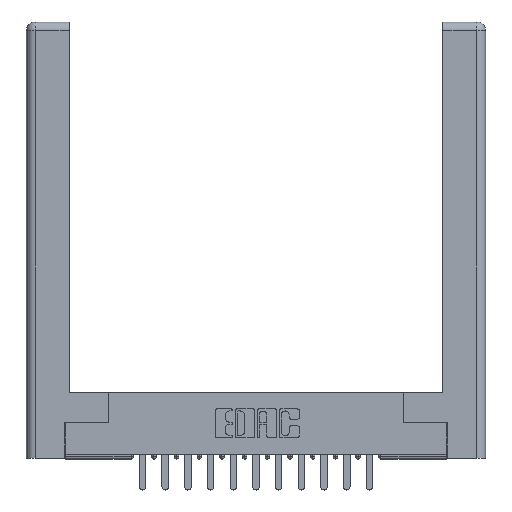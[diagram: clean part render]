
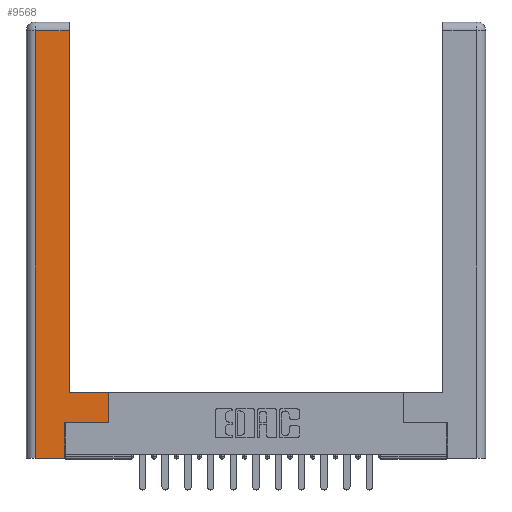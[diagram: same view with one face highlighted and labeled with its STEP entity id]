
A CAD part, top view. The second image highlights one B-rep face of the part: STEP entity #9568.
In plain terms, the highlighted planar face has unit normal (0, 0, 1).
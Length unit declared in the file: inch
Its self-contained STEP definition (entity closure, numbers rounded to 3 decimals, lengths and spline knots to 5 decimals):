
#26 = LINE ( 'NONE', #1676, #1775 ) ;
#109 = VECTOR ( 'NONE', #3716, 39.37008 ) ;
#846 = VERTEX_POINT ( 'NONE', #5462 ) ;
#1676 = CARTESIAN_POINT ( 'NONE',  ( 0.265, 0.245, 0. ) ) ;
#1759 = CARTESIAN_POINT ( 'NONE',  ( 0.565, 0.45, 0. ) ) ;
#1775 = VECTOR ( 'NONE', #3091, 39.37008 ) ;
#1989 = VERTEX_POINT ( 'NONE', #14315 ) ;
#2043 = CARTESIAN_POINT ( 'NONE',  ( 0., 0., 0. ) ) ;
#2630 = LINE ( 'NONE', #7723, #7914 ) ;
#3040 = EDGE_LOOP ( 'NONE', ( #3191, #3085, #13605, #9884, #14091, #15902, #15129, #17615 ) ) ;
#3085 = ORIENTED_EDGE ( 'NONE', *, *, #5495, .T. ) ;
#3091 = DIRECTION ( 'NONE',  ( 0., 1., 0. ) ) ;
#3191 = ORIENTED_EDGE ( 'NONE', *, *, #6668, .T. ) ;
#3481 = VECTOR ( 'NONE', #5031, 39.37008 ) ;
#3716 = DIRECTION ( 'NONE',  ( 0., 1., 0. ) ) ;
#4754 = VECTOR ( 'NONE', #14492, 39.37008 ) ;
#5031 = DIRECTION ( 'NONE',  ( 0., 1., 0. ) ) ;
#5462 = CARTESIAN_POINT ( 'NONE',  ( 0.565, 0.45, 0. ) ) ;
#5495 = EDGE_CURVE ( 'NONE', #13693, #15937, #8516, .T. ) ;
#5678 = LINE ( 'NONE', #1759, #3481 ) ;
#5957 = DIRECTION ( 'NONE',  ( 1., 0., 0. ) ) ;
#6668 = EDGE_CURVE ( 'NONE', #15772, #13693, #15689, .T. ) ;
#6738 = CARTESIAN_POINT ( 'NONE',  ( 0.265, 0., 0. ) ) ;
#7490 = CARTESIAN_POINT ( 'NONE',  ( 0.0615, 2.94, 0. ) ) ;
#7723 = CARTESIAN_POINT ( 'NONE',  ( 0.265, 0., 0. ) ) ;
#7733 = CARTESIAN_POINT ( 'NONE',  ( 0.295, 3., 0. ) ) ;
#7769 = DIRECTION ( 'NONE',  ( 0., 0., -1. ) ) ;
#7914 = VECTOR ( 'NONE', #17553, 39.37008 ) ;
#7922 = CARTESIAN_POINT ( 'NONE',  ( 0.0615, 2.94, 0. ) ) ;
#7933 = VERTEX_POINT ( 'NONE', #6738 ) ;
#8221 = LINE ( 'NONE', #10044, #15889 ) ;
#8516 = LINE ( 'NONE', #7490, #4754 ) ;
#8743 = DIRECTION ( 'NONE',  ( -1., 0., 0. ) ) ;
#9003 = CARTESIAN_POINT ( 'NONE',  ( 0.0615, 0., 0. ) ) ;
#9471 = LINE ( 'NONE', #9003, #13603 ) ;
#9568 = ADVANCED_FACE ( 'NONE', ( #13273 ), #11882, .F. ) ;
#9676 = CARTESIAN_POINT ( 'NONE',  ( 0.0615, 0., 0. ) ) ;
#9677 = VERTEX_POINT ( 'NONE', #16522 ) ;
#9884 = ORIENTED_EDGE ( 'NONE', *, *, #14721, .T. ) ;
#9958 = EDGE_CURVE ( 'NONE', #9677, #1989, #17436, .T. ) ;
#9999 = VECTOR ( 'NONE', #5957, 39.37008 ) ;
#10044 = CARTESIAN_POINT ( 'NONE',  ( 0.295, 0.45, 0. ) ) ;
#10617 = EDGE_CURVE ( 'NONE', #7933, #9677, #26, .T. ) ;
#11488 = CARTESIAN_POINT ( 'NONE',  ( 0.565, 0.245, 0. ) ) ;
#11720 = DIRECTION ( 'NONE',  ( 0., -1., 0. ) ) ;
#11882 = PLANE ( 'NONE',  #13489 ) ;
#12344 = EDGE_CURVE ( 'NONE', #15937, #12749, #9471, .T. ) ;
#12749 = VERTEX_POINT ( 'NONE', #9676 ) ;
#13273 = FACE_OUTER_BOUND ( 'NONE', #3040, .T. ) ;
#13489 = AXIS2_PLACEMENT_3D ( 'NONE', #2043, #7769, #15927 ) ;
#13603 = VECTOR ( 'NONE', #11720, 39.37008 ) ;
#13605 = ORIENTED_EDGE ( 'NONE', *, *, #12344, .T. ) ;
#13693 = VERTEX_POINT ( 'NONE', #16582 ) ;
#14003 = EDGE_CURVE ( 'NONE', #846, #15772, #8221, .T. ) ;
#14091 = ORIENTED_EDGE ( 'NONE', *, *, #10617, .T. ) ;
#14315 = CARTESIAN_POINT ( 'NONE',  ( 0.565, 0.245, 0. ) ) ;
#14492 = DIRECTION ( 'NONE',  ( -1., 0., 0. ) ) ;
#14721 = EDGE_CURVE ( 'NONE', #12749, #7933, #2630, .T. ) ;
#15129 = ORIENTED_EDGE ( 'NONE', *, *, #15356, .T. ) ;
#15356 = EDGE_CURVE ( 'NONE', #1989, #846, #5678, .T. ) ;
#15689 = LINE ( 'NONE', #7733, #109 ) ;
#15772 = VERTEX_POINT ( 'NONE', #17711 ) ;
#15889 = VECTOR ( 'NONE', #8743, 39.37008 ) ;
#15902 = ORIENTED_EDGE ( 'NONE', *, *, #9958, .T. ) ;
#15927 = DIRECTION ( 'NONE',  ( -1., 0., 0. ) ) ;
#15937 = VERTEX_POINT ( 'NONE', #7922 ) ;
#16522 = CARTESIAN_POINT ( 'NONE',  ( 0.265, 0.245, 0. ) ) ;
#16582 = CARTESIAN_POINT ( 'NONE',  ( 0.295, 2.94, 0. ) ) ;
#17436 = LINE ( 'NONE', #11488, #9999 ) ;
#17553 = DIRECTION ( 'NONE',  ( 1., 0., 0. ) ) ;
#17615 = ORIENTED_EDGE ( 'NONE', *, *, #14003, .T. ) ;
#17711 = CARTESIAN_POINT ( 'NONE',  ( 0.295, 0.45, 0. ) ) ;
